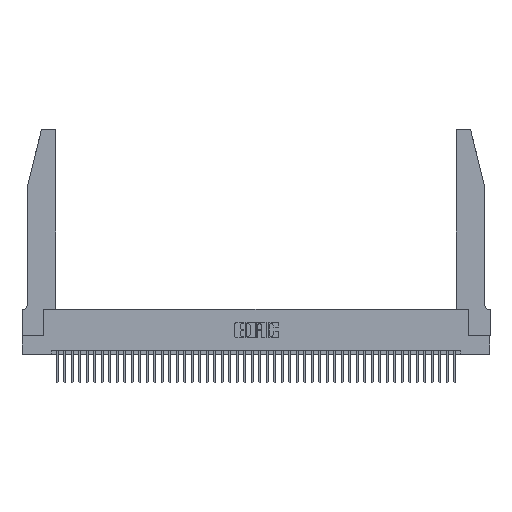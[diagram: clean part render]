
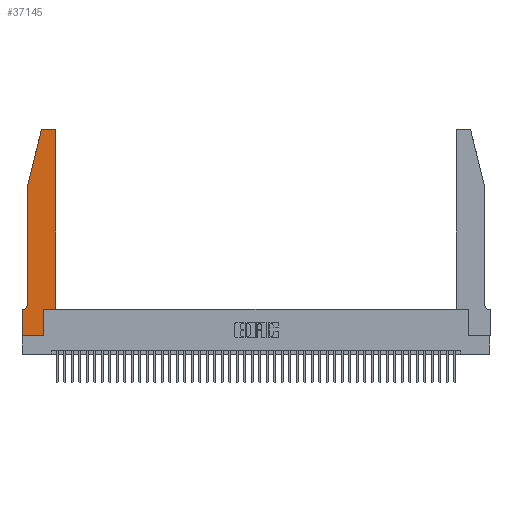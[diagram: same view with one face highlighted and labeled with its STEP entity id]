
A CAD part, top view. The second image highlights one B-rep face of the part: STEP entity #37145.
In plain terms, the highlighted planar face has unit normal (0, 0, 1).
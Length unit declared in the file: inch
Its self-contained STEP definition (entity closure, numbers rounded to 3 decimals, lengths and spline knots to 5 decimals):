
#66 = CARTESIAN_POINT ( 'NONE',  ( 0.284, 2.75, 0.37 ) ) ;
#1951 = VECTOR ( 'NONE', #14868, 39.37008 ) ;
#2356 = CARTESIAN_POINT ( 'NONE',  ( 0.25487, 2.72718, 0.37 ) ) ;
#2482 = ORIENTED_EDGE ( 'NONE', *, *, #10367, .T. ) ;
#2812 = ORIENTED_EDGE ( 'NONE', *, *, #25958, .T. ) ;
#2912 = LINE ( 'NONE', #37780, #20716 ) ;
#3262 = VERTEX_POINT ( 'NONE', #22737 ) ;
#3421 = DIRECTION ( 'NONE',  ( 1., 0., 0. ) ) ;
#5265 = LINE ( 'NONE', #26335, #23038 ) ;
#5453 = VERTEX_POINT ( 'NONE', #27438 ) ;
#6029 = CARTESIAN_POINT ( 'NONE',  ( 0.284, 2.72, 0.37 ) ) ;
#7570 = ORIENTED_EDGE ( 'NONE', *, *, #24217, .T. ) ;
#8140 = VECTOR ( 'NONE', #24084, 39.37008 ) ;
#8898 = VECTOR ( 'NONE', #31074, 39.37008 ) ;
#9403 = ORIENTED_EDGE ( 'NONE', *, *, #35600, .T. ) ;
#9664 = DIRECTION ( 'NONE',  ( 1., 0., 0. ) ) ;
#10018 = CARTESIAN_POINT ( 'NONE',  ( 0., 0.35, 0.37 ) ) ;
#10159 = ORIENTED_EDGE ( 'NONE', *, *, #26770, .T. ) ;
#10367 = EDGE_CURVE ( 'NONE', #3262, #12718, #29722, .T. ) ;
#11297 = CARTESIAN_POINT ( 'NONE',  ( 0.2865, 0.35, 0.37 ) ) ;
#11520 = EDGE_CURVE ( 'NONE', #24057, #36517, #45390, .T. ) ;
#12718 = VERTEX_POINT ( 'NONE', #44501 ) ;
#13374 = DIRECTION ( 'NONE',  ( 1., 0., 0. ) ) ;
#13562 = DIRECTION ( 'NONE',  ( 0., 0., 1. ) ) ;
#13625 = DIRECTION ( 'NONE',  ( 0., 0., 1. ) ) ;
#13791 = CARTESIAN_POINT ( 'NONE',  ( 0.0755, 0.35, 0.37 ) ) ;
#14297 = CIRCLE ( 'NONE', #16160, 0.07 ) ;
#14868 = DIRECTION ( 'NONE',  ( 0., 1., 0. ) ) ;
#15260 = CARTESIAN_POINT ( 'NONE',  ( 0.4505, 2.72, 0.37 ) ) ;
#16160 = AXIS2_PLACEMENT_3D ( 'NONE', #16411, #40821, #19929 ) ;
#16411 = CARTESIAN_POINT ( 'NONE',  ( 0.0055, 0.42, 0.37 ) ) ;
#16629 = EDGE_CURVE ( 'NONE', #37818, #3262, #30155, .T. ) ;
#17242 = CARTESIAN_POINT ( 'NONE',  ( 0.2865, 0., 0.37 ) ) ;
#17457 = VERTEX_POINT ( 'NONE', #15260 ) ;
#18200 = LINE ( 'NONE', #34299, #43805 ) ;
#18964 = AXIS2_PLACEMENT_3D ( 'NONE', #34464, #13562, #37961 ) ;
#19929 = DIRECTION ( 'NONE',  ( -1., 0., 0. ) ) ;
#20623 = AXIS2_PLACEMENT_3D ( 'NONE', #6029, #30715, #9664 ) ;
#20716 = VECTOR ( 'NONE', #23965, 39.37008 ) ;
#20980 = VERTEX_POINT ( 'NONE', #22700 ) ;
#21147 = CARTESIAN_POINT ( 'NONE',  ( 0.4505, 0.35, 0.37 ) ) ;
#21675 = ORIENTED_EDGE ( 'NONE', *, *, #31850, .T. ) ;
#21830 = LINE ( 'NONE', #30829, #39232 ) ;
#22489 = CIRCLE ( 'NONE', #18964, 0.03 ) ;
#22531 = VERTEX_POINT ( 'NONE', #42292 ) ;
#22573 = CARTESIAN_POINT ( 'NONE',  ( 0., 0.35, 0.37 ) ) ;
#22700 = CARTESIAN_POINT ( 'NONE',  ( 0.0055, 0.35, 0.37 ) ) ;
#22737 = CARTESIAN_POINT ( 'NONE',  ( 0.2865, 0.35, 0.37 ) ) ;
#23038 = VECTOR ( 'NONE', #29821, 39.37008 ) ;
#23338 = ORIENTED_EDGE ( 'NONE', *, *, #32389, .T. ) ;
#23962 = DIRECTION ( 'NONE',  ( 0., 1., 0. ) ) ;
#23965 = DIRECTION ( 'NONE',  ( 0., -1., 0. ) ) ;
#24057 = VERTEX_POINT ( 'NONE', #2356 ) ;
#24084 = DIRECTION ( 'NONE',  ( -0.239, -0.971, 0. ) ) ;
#24217 = EDGE_CURVE ( 'NONE', #20980, #35994, #27610, .T. ) ;
#24504 = ORIENTED_EDGE ( 'NONE', *, *, #32385, .T. ) ;
#25958 = EDGE_CURVE ( 'NONE', #35994, #5453, #29631, .T. ) ;
#26335 = CARTESIAN_POINT ( 'NONE',  ( 0.2605, 2.75, 0.37 ) ) ;
#26770 = EDGE_CURVE ( 'NONE', #17457, #22531, #22489, .T. ) ;
#27436 = VECTOR ( 'NONE', #43488, 39.37008 ) ;
#27438 = CARTESIAN_POINT ( 'NONE',  ( 0., 0., 0.37 ) ) ;
#27529 = VECTOR ( 'NONE', #3421, 39.37008 ) ;
#27610 = LINE ( 'NONE', #13791, #8898 ) ;
#28227 = ORIENTED_EDGE ( 'NONE', *, *, #41835, .T. ) ;
#29631 = LINE ( 'NONE', #32882, #27436 ) ;
#29722 = LINE ( 'NONE', #21147, #27529 ) ;
#29808 = ORIENTED_EDGE ( 'NONE', *, *, #16629, .T. ) ;
#29821 = DIRECTION ( 'NONE',  ( -1., 0., 0. ) ) ;
#29923 = ORIENTED_EDGE ( 'NONE', *, *, #30800, .T. ) ;
#30155 = LINE ( 'NONE', #11297, #1951 ) ;
#30715 = DIRECTION ( 'NONE',  ( 0., 0., 1. ) ) ;
#30800 = EDGE_CURVE ( 'NONE', #38691, #20980, #14297, .T. ) ;
#30829 = CARTESIAN_POINT ( 'NONE',  ( 0., 0., 0.37 ) ) ;
#31060 = PLANE ( 'NONE',  #33309 ) ;
#31074 = DIRECTION ( 'NONE',  ( -1., 0., 0. ) ) ;
#31850 = EDGE_CURVE ( 'NONE', #39747, #24057, #34372, .T. ) ;
#32078 = FACE_OUTER_BOUND ( 'NONE', #44073, .T. ) ;
#32116 = CARTESIAN_POINT ( 'NONE',  ( 0.0755, 2., 0.37 ) ) ;
#32385 = EDGE_CURVE ( 'NONE', #5453, #37818, #21830, .T. ) ;
#32389 = EDGE_CURVE ( 'NONE', #36517, #38691, #2912, .T. ) ;
#32760 = CARTESIAN_POINT ( 'NONE',  ( 0.0755, 0.42, 0.37 ) ) ;
#32882 = CARTESIAN_POINT ( 'NONE',  ( 0., 0., 0.37 ) ) ;
#33309 = AXIS2_PLACEMENT_3D ( 'NONE', #10018, #13625, #38019 ) ;
#33626 = ORIENTED_EDGE ( 'NONE', *, *, #11520, .T. ) ;
#34299 = CARTESIAN_POINT ( 'NONE',  ( 0.4505, 0.35, 0.37 ) ) ;
#34372 = CIRCLE ( 'NONE', #20623, 0.03 ) ;
#34464 = CARTESIAN_POINT ( 'NONE',  ( 0.4205, 2.72, 0.37 ) ) ;
#35600 = EDGE_CURVE ( 'NONE', #12718, #17457, #18200, .T. ) ;
#35994 = VERTEX_POINT ( 'NONE', #22573 ) ;
#36517 = VERTEX_POINT ( 'NONE', #32116 ) ;
#37145 = ADVANCED_FACE ( 'NONE', ( #32078 ), #31060, .T. ) ;
#37780 = CARTESIAN_POINT ( 'NONE',  ( 0.0755, 2., 0.37 ) ) ;
#37818 = VERTEX_POINT ( 'NONE', #17242 ) ;
#37961 = DIRECTION ( 'NONE',  ( 1., 0., 0. ) ) ;
#38019 = DIRECTION ( 'NONE',  ( 1., 0., 0. ) ) ;
#38691 = VERTEX_POINT ( 'NONE', #32760 ) ;
#39232 = VECTOR ( 'NONE', #13374, 39.37008 ) ;
#39747 = VERTEX_POINT ( 'NONE', #66 ) ;
#40821 = DIRECTION ( 'NONE',  ( 0., 0., -1. ) ) ;
#41415 = CARTESIAN_POINT ( 'NONE',  ( 0.0755, 2., 0.37 ) ) ;
#41835 = EDGE_CURVE ( 'NONE', #22531, #39747, #5265, .T. ) ;
#42292 = CARTESIAN_POINT ( 'NONE',  ( 0.4205, 2.75, 0.37 ) ) ;
#43488 = DIRECTION ( 'NONE',  ( 0., -1., 0. ) ) ;
#43805 = VECTOR ( 'NONE', #23962, 39.37008 ) ;
#44073 = EDGE_LOOP ( 'NONE', ( #28227, #21675, #33626, #23338, #29923, #7570, #2812, #24504, #29808, #2482, #9403, #10159 ) ) ;
#44501 = CARTESIAN_POINT ( 'NONE',  ( 0.4505, 0.35, 0.37 ) ) ;
#45390 = LINE ( 'NONE', #41415, #8140 ) ;
